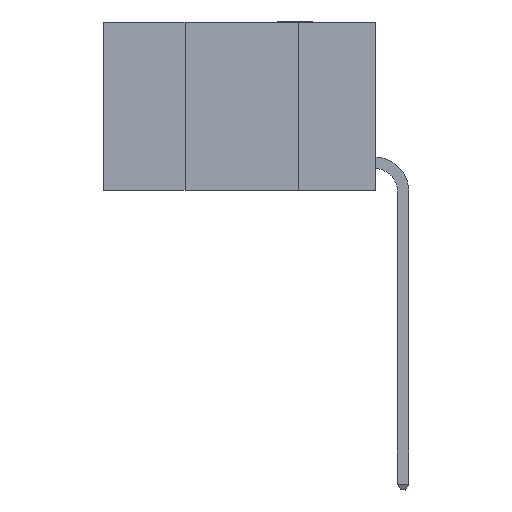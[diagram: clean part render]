
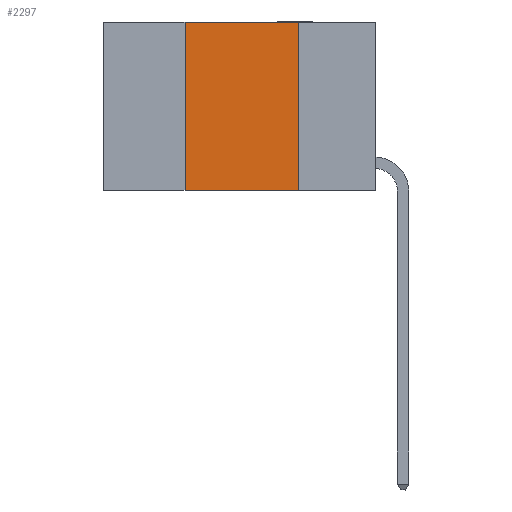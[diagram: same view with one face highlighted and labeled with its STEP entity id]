
A CAD part, left-side view. The second image highlights one B-rep face of the part: STEP entity #2297.
In plain terms, the highlighted planar face has unit normal (-1, 0, 0).
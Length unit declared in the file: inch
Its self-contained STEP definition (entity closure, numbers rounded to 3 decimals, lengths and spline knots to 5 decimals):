
#1098 = LINE ( 'NONE', #5315, #12915 ) ;
#1566 = EDGE_CURVE ( 'NONE', #10237, #9861, #1098, .T. ) ;
#1713 = DIRECTION ( 'NONE',  ( 1., 0., 0. ) ) ;
#1817 = CARTESIAN_POINT ( 'NONE',  ( 0., 0.17, 0. ) ) ;
#2297 = ADVANCED_FACE ( 'NONE', ( #8695 ), #13043, .F. ) ;
#2573 = CARTESIAN_POINT ( 'NONE',  ( 0., 0.42, -0.37 ) ) ;
#3019 = LINE ( 'NONE', #12358, #5766 ) ;
#3046 = DIRECTION ( 'NONE',  ( 0., 0., -1. ) ) ;
#3067 = CARTESIAN_POINT ( 'NONE',  ( 0., 0.42, 0. ) ) ;
#3807 = VECTOR ( 'NONE', #3046, 39.37008 ) ;
#4673 = ORIENTED_EDGE ( 'NONE', *, *, #7411, .F. ) ;
#4787 = LINE ( 'NONE', #3067, #8050 ) ;
#5176 = VERTEX_POINT ( 'NONE', #8122 ) ;
#5299 = VERTEX_POINT ( 'NONE', #2573 ) ;
#5315 = CARTESIAN_POINT ( 'NONE',  ( 0., 0.6, 0. ) ) ;
#5722 = DIRECTION ( 'NONE',  ( 0., -1., 0. ) ) ;
#5766 = VECTOR ( 'NONE', #5722, 39.37008 ) ;
#6283 = EDGE_LOOP ( 'NONE', ( #4673, #7927, #11231, #14583 ) ) ;
#6536 = EDGE_CURVE ( 'NONE', #5299, #10237, #4787, .T. ) ;
#7171 = CARTESIAN_POINT ( 'NONE',  ( 0., 0.42, 0. ) ) ;
#7411 = EDGE_CURVE ( 'NONE', #9861, #5176, #9759, .T. ) ;
#7480 = AXIS2_PLACEMENT_3D ( 'NONE', #8617, #1713, #9734 ) ;
#7927 = ORIENTED_EDGE ( 'NONE', *, *, #1566, .F. ) ;
#8050 = VECTOR ( 'NONE', #8727, 39.37008 ) ;
#8122 = CARTESIAN_POINT ( 'NONE',  ( 0., 0.17, -0.37 ) ) ;
#8617 = CARTESIAN_POINT ( 'NONE',  ( 0., 0.6, 0. ) ) ;
#8649 = DIRECTION ( 'NONE',  ( 0., -1., 0. ) ) ;
#8695 = FACE_OUTER_BOUND ( 'NONE', #6283, .T. ) ;
#8727 = DIRECTION ( 'NONE',  ( 0., 0., 1. ) ) ;
#9734 = DIRECTION ( 'NONE',  ( 0., 0., -1. ) ) ;
#9759 = LINE ( 'NONE', #1817, #3807 ) ;
#9861 = VERTEX_POINT ( 'NONE', #11100 ) ;
#10237 = VERTEX_POINT ( 'NONE', #7171 ) ;
#11100 = CARTESIAN_POINT ( 'NONE',  ( 0., 0.17, 0. ) ) ;
#11231 = ORIENTED_EDGE ( 'NONE', *, *, #6536, .F. ) ;
#12358 = CARTESIAN_POINT ( 'NONE',  ( 0., 0.6, -0.37 ) ) ;
#12748 = EDGE_CURVE ( 'NONE', #5299, #5176, #3019, .T. ) ;
#12915 = VECTOR ( 'NONE', #8649, 39.37008 ) ;
#13043 = PLANE ( 'NONE',  #7480 ) ;
#14583 = ORIENTED_EDGE ( 'NONE', *, *, #12748, .T. ) ;
